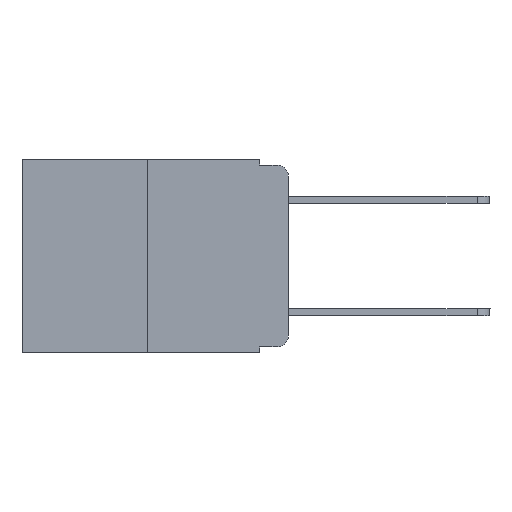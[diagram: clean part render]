
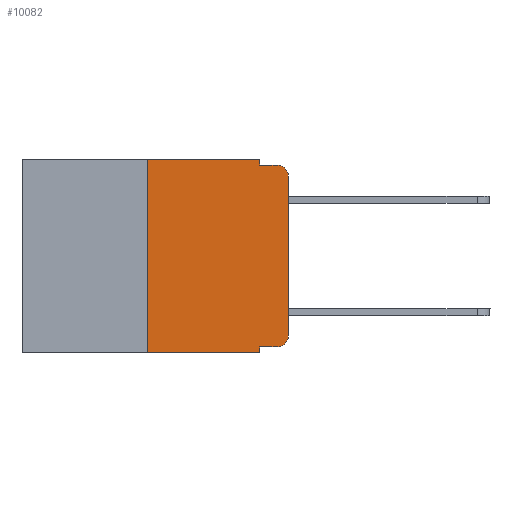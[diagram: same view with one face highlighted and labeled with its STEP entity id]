
A CAD part, left-side view. The second image highlights one B-rep face of the part: STEP entity #10082.
In plain terms, the highlighted planar face has unit normal (-1, 0, 0).
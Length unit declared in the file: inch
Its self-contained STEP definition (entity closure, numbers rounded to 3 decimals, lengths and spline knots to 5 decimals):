
#99 = CARTESIAN_POINT ( 'NONE',  ( 0., 0.051, -0.333 ) ) ;
#212 = ORIENTED_EDGE ( 'NONE', *, *, #8209, .T. ) ;
#279 = DIRECTION ( 'NONE',  ( 0., 0., -1. ) ) ;
#568 = VERTEX_POINT ( 'NONE', #4682 ) ;
#918 = LINE ( 'NONE', #8428, #3016 ) ;
#998 = VECTOR ( 'NONE', #6622, 39.37008 ) ;
#1133 = LINE ( 'NONE', #12793, #2682 ) ;
#1230 = ORIENTED_EDGE ( 'NONE', *, *, #12556, .F. ) ;
#1335 = AXIS2_PLACEMENT_3D ( 'NONE', #5727, #6859, #7974 ) ;
#1458 = CARTESIAN_POINT ( 'NONE',  ( 0., 0.02, -0.333 ) ) ;
#1525 = LINE ( 'NONE', #14231, #998 ) ;
#2212 = CARTESIAN_POINT ( 'NONE',  ( 0., 0.051, 0. ) ) ;
#2432 = LINE ( 'NONE', #99, #10040 ) ;
#2444 = PLANE ( 'NONE',  #1335 ) ;
#2682 = VECTOR ( 'NONE', #13845, 39.37008 ) ;
#3016 = VECTOR ( 'NONE', #10442, 39.37008 ) ;
#3436 = ORIENTED_EDGE ( 'NONE', *, *, #10263, .F. ) ;
#3475 = EDGE_CURVE ( 'NONE', #8584, #6125, #12457, .T. ) ;
#3487 = ORIENTED_EDGE ( 'NONE', *, *, #11660, .T. ) ;
#3594 = CARTESIAN_POINT ( 'NONE',  ( 0., 0.25, -0.343 ) ) ;
#3988 = VERTEX_POINT ( 'NONE', #1458 ) ;
#4308 = CARTESIAN_POINT ( 'NONE',  ( 0., 0.02, -0.03 ) ) ;
#4549 = VERTEX_POINT ( 'NONE', #12307 ) ;
#4682 = CARTESIAN_POINT ( 'NONE',  ( 0., 0.02, -0.01 ) ) ;
#5017 = CARTESIAN_POINT ( 'NONE',  ( 0., 0., -0.03 ) ) ;
#5290 = VECTOR ( 'NONE', #14165, 39.37008 ) ;
#5339 = CARTESIAN_POINT ( 'NONE',  ( 0., 0.051, -0.333 ) ) ;
#5482 = VECTOR ( 'NONE', #10221, 39.37008 ) ;
#5508 = VERTEX_POINT ( 'NONE', #9817 ) ;
#5533 = EDGE_CURVE ( 'NONE', #5855, #568, #13468, .T. ) ;
#5712 = AXIS2_PLACEMENT_3D ( 'NONE', #6964, #12540, #279 ) ;
#5727 = CARTESIAN_POINT ( 'NONE',  ( 0., 0.473, 0. ) ) ;
#5855 = VERTEX_POINT ( 'NONE', #5017 ) ;
#6093 = EDGE_CURVE ( 'NONE', #11853, #10863, #1525, .T. ) ;
#6125 = VERTEX_POINT ( 'NONE', #2212 ) ;
#6166 = LINE ( 'NONE', #6454, #5290 ) ;
#6454 = CARTESIAN_POINT ( 'NONE',  ( 0., 0.473, -0.343 ) ) ;
#6589 = DIRECTION ( 'NONE',  ( 0., 0., -1. ) ) ;
#6622 = DIRECTION ( 'NONE',  ( 0., 0., -1. ) ) ;
#6859 = DIRECTION ( 'NONE',  ( 1., 0., 0. ) ) ;
#6964 = CARTESIAN_POINT ( 'NONE',  ( 0., 0.02, -0.313 ) ) ;
#7043 = CARTESIAN_POINT ( 'NONE',  ( 0., 0.25, 0. ) ) ;
#7871 = EDGE_LOOP ( 'NONE', ( #3487, #8360, #1230, #8826, #8767, #3436, #9003, #13042, #212, #11276 ) ) ;
#7964 = CARTESIAN_POINT ( 'NONE',  ( 0., 0.473, 0. ) ) ;
#7974 = DIRECTION ( 'NONE',  ( 0., 0., -1. ) ) ;
#8169 = AXIS2_PLACEMENT_3D ( 'NONE', #4308, #13184, #6589 ) ;
#8208 = CIRCLE ( 'NONE', #5712, 0.02 ) ;
#8209 = EDGE_CURVE ( 'NONE', #11853, #3988, #2432, .T. ) ;
#8360 = ORIENTED_EDGE ( 'NONE', *, *, #5533, .T. ) ;
#8410 = CARTESIAN_POINT ( 'NONE',  ( 0., 0.25, 0. ) ) ;
#8428 = CARTESIAN_POINT ( 'NONE',  ( 0., 0.051, -0.01 ) ) ;
#8584 = VERTEX_POINT ( 'NONE', #8410 ) ;
#8767 = ORIENTED_EDGE ( 'NONE', *, *, #3475, .F. ) ;
#8826 = ORIENTED_EDGE ( 'NONE', *, *, #11858, .F. ) ;
#8986 = DIRECTION ( 'NONE',  ( 0., -1., 0. ) ) ;
#9003 = ORIENTED_EDGE ( 'NONE', *, *, #10535, .T. ) ;
#9138 = FACE_OUTER_BOUND ( 'NONE', #7871, .T. ) ;
#9262 = CARTESIAN_POINT ( 'NONE',  ( 0., 0.051, -0.343 ) ) ;
#9539 = VECTOR ( 'NONE', #8986, 39.37008 ) ;
#9817 = CARTESIAN_POINT ( 'NONE',  ( 0., 0.051, -0.01 ) ) ;
#9848 = CARTESIAN_POINT ( 'NONE',  ( 0., 0.051, 0. ) ) ;
#9946 = DIRECTION ( 'NONE',  ( 0., -1., 0. ) ) ;
#10040 = VECTOR ( 'NONE', #9946, 39.37008 ) ;
#10082 = ADVANCED_FACE ( 'NONE', ( #9138 ), #2444, .F. ) ;
#10221 = DIRECTION ( 'NONE',  ( 0., 0., 1. ) ) ;
#10263 = EDGE_CURVE ( 'NONE', #12300, #8584, #13091, .T. ) ;
#10442 = DIRECTION ( 'NONE',  ( 0., -1., 0. ) ) ;
#10535 = EDGE_CURVE ( 'NONE', #12300, #10863, #6166, .T. ) ;
#10807 = LINE ( 'NONE', #9848, #12885 ) ;
#10863 = VERTEX_POINT ( 'NONE', #9262 ) ;
#11276 = ORIENTED_EDGE ( 'NONE', *, *, #13001, .T. ) ;
#11660 = EDGE_CURVE ( 'NONE', #4549, #5855, #1133, .T. ) ;
#11853 = VERTEX_POINT ( 'NONE', #5339 ) ;
#11858 = EDGE_CURVE ( 'NONE', #6125, #5508, #10807, .T. ) ;
#12053 = DIRECTION ( 'NONE',  ( 0., 0., -1. ) ) ;
#12300 = VERTEX_POINT ( 'NONE', #3594 ) ;
#12307 = CARTESIAN_POINT ( 'NONE',  ( 0., 0., -0.313 ) ) ;
#12457 = LINE ( 'NONE', #7964, #9539 ) ;
#12540 = DIRECTION ( 'NONE',  ( -1., 0., 0. ) ) ;
#12556 = EDGE_CURVE ( 'NONE', #5508, #568, #918, .T. ) ;
#12793 = CARTESIAN_POINT ( 'NONE',  ( 0., 0., 0. ) ) ;
#12885 = VECTOR ( 'NONE', #12053, 39.37008 ) ;
#13001 = EDGE_CURVE ( 'NONE', #3988, #4549, #8208, .T. ) ;
#13042 = ORIENTED_EDGE ( 'NONE', *, *, #6093, .F. ) ;
#13091 = LINE ( 'NONE', #7043, #5482 ) ;
#13184 = DIRECTION ( 'NONE',  ( -1., 0., 0. ) ) ;
#13468 = CIRCLE ( 'NONE', #8169, 0.02 ) ;
#13845 = DIRECTION ( 'NONE',  ( 0., 0., 1. ) ) ;
#14165 = DIRECTION ( 'NONE',  ( 0., -1., 0. ) ) ;
#14231 = CARTESIAN_POINT ( 'NONE',  ( 0., 0.051, 0. ) ) ;
